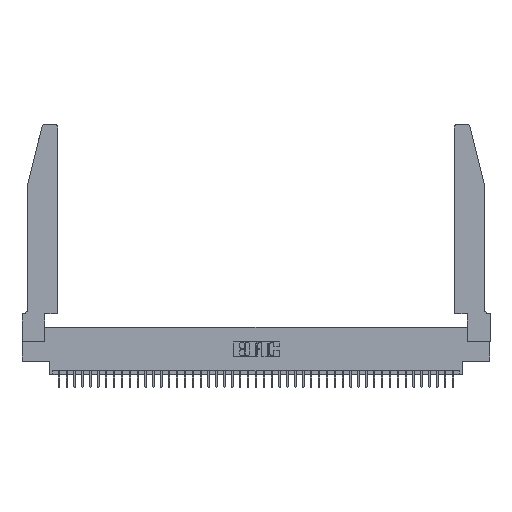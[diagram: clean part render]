
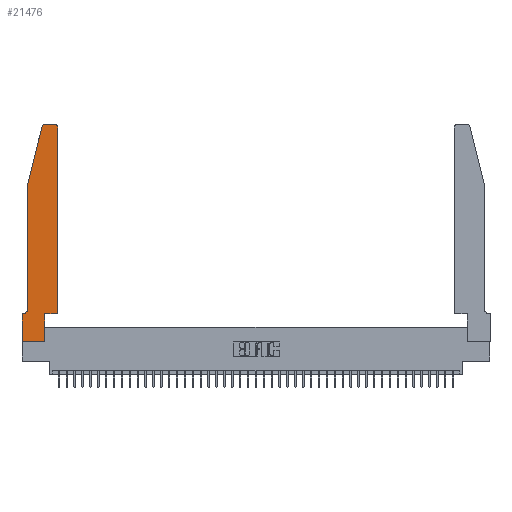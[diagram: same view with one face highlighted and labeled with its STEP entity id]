
A CAD part, top view. The second image highlights one B-rep face of the part: STEP entity #21476.
In plain terms, the highlighted planar face has unit normal (0, 0, 1).
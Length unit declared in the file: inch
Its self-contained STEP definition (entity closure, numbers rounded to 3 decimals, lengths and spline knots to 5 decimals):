
#201 = CARTESIAN_POINT ( 'NONE',  ( 0., 0.35, 0.37 ) ) ;
#630 = FACE_OUTER_BOUND ( 'NONE', #7524, .T. ) ;
#2480 = CARTESIAN_POINT ( 'NONE',  ( 0.4505, 0.35, 0.37 ) ) ;
#2744 = CARTESIAN_POINT ( 'NONE',  ( 0.0755, 2., 0.37 ) ) ;
#3392 = VECTOR ( 'NONE', #34415, 39.37008 ) ;
#3431 = VERTEX_POINT ( 'NONE', #37091 ) ;
#3990 = DIRECTION ( 'NONE',  ( 0., 1., 0. ) ) ;
#4061 = ORIENTED_EDGE ( 'NONE', *, *, #27604, .T. ) ;
#4428 = CARTESIAN_POINT ( 'NONE',  ( 0.4205, 2.75, 0.37 ) ) ;
#4953 = EDGE_CURVE ( 'NONE', #30414, #35835, #20170, .T. ) ;
#5195 = AXIS2_PLACEMENT_3D ( 'NONE', #39839, #42639, #13471 ) ;
#5774 = VECTOR ( 'NONE', #9943, 39.37008 ) ;
#6065 = VECTOR ( 'NONE', #11434, 39.37008 ) ;
#6273 = CARTESIAN_POINT ( 'NONE',  ( 0.2605, 2.75, 0.37 ) ) ;
#6941 = DIRECTION ( 'NONE',  ( 0., 0., 1. ) ) ;
#7218 = PLANE ( 'NONE',  #25998 ) ;
#7524 = EDGE_LOOP ( 'NONE', ( #34817, #4061, #43095, #39921, #35769, #30388, #33213, #10723, #20108, #25203, #20987, #14579 ) ) ;
#7546 = VERTEX_POINT ( 'NONE', #34997 ) ;
#8217 = LINE ( 'NONE', #36233, #42157 ) ;
#8268 = CARTESIAN_POINT ( 'NONE',  ( 0.4505, 2.72, 0.37 ) ) ;
#8286 = CIRCLE ( 'NONE', #5195, 0.03 ) ;
#9338 = DIRECTION ( 'NONE',  ( 0., 0., -1. ) ) ;
#9943 = DIRECTION ( 'NONE',  ( -0.239, -0.971, 0. ) ) ;
#10118 = VERTEX_POINT ( 'NONE', #12332 ) ;
#10639 = DIRECTION ( 'NONE',  ( 0., 1., 0. ) ) ;
#10723 = ORIENTED_EDGE ( 'NONE', *, *, #36089, .T. ) ;
#10824 = VERTEX_POINT ( 'NONE', #27825 ) ;
#11266 = CARTESIAN_POINT ( 'NONE',  ( 0.4505, 0.35, 0.37 ) ) ;
#11434 = DIRECTION ( 'NONE',  ( 0., -1., 0. ) ) ;
#11556 = LINE ( 'NONE', #6273, #28538 ) ;
#12150 = VERTEX_POINT ( 'NONE', #41210 ) ;
#12332 = CARTESIAN_POINT ( 'NONE',  ( 0.0755, 2., 0.37 ) ) ;
#12453 = EDGE_CURVE ( 'NONE', #40874, #32101, #20290, .T. ) ;
#13342 = CARTESIAN_POINT ( 'NONE',  ( 0.284, 2.75, 0.37 ) ) ;
#13358 = VECTOR ( 'NONE', #3990, 39.37008 ) ;
#13471 = DIRECTION ( 'NONE',  ( 1., 0., 0. ) ) ;
#14579 = ORIENTED_EDGE ( 'NONE', *, *, #4953, .T. ) ;
#15355 = EDGE_CURVE ( 'NONE', #35835, #32494, #11556, .T. ) ;
#15443 = VERTEX_POINT ( 'NONE', #24519 ) ;
#15636 = DIRECTION ( 'NONE',  ( -1., 0., 0. ) ) ;
#16541 = DIRECTION ( 'NONE',  ( -1., 0., 0. ) ) ;
#17772 = EDGE_CURVE ( 'NONE', #12150, #7546, #37866, .T. ) ;
#19574 = DIRECTION ( 'NONE',  ( 0., 0., 1. ) ) ;
#20108 = ORIENTED_EDGE ( 'NONE', *, *, #32672, .T. ) ;
#20170 = CIRCLE ( 'NONE', #40223, 0.03 ) ;
#20290 = CIRCLE ( 'NONE', #42739, 0.07 ) ;
#20987 = ORIENTED_EDGE ( 'NONE', *, *, #30800, .T. ) ;
#21420 = CARTESIAN_POINT ( 'NONE',  ( 0., 0., 0.37 ) ) ;
#21476 = ADVANCED_FACE ( 'NONE', ( #630 ), #7218, .T. ) ;
#22275 = EDGE_CURVE ( 'NONE', #3431, #10118, #37080, .T. ) ;
#23863 = CARTESIAN_POINT ( 'NONE',  ( 0.4505, 0.35, 0.37 ) ) ;
#24519 = CARTESIAN_POINT ( 'NONE',  ( 0.2865, 0., 0.37 ) ) ;
#25106 = CARTESIAN_POINT ( 'NONE',  ( 0.0055, 0.35, 0.37 ) ) ;
#25203 = ORIENTED_EDGE ( 'NONE', *, *, #31127, .T. ) ;
#25998 = AXIS2_PLACEMENT_3D ( 'NONE', #201, #6941, #27710 ) ;
#27604 = EDGE_CURVE ( 'NONE', #32494, #3431, #8286, .T. ) ;
#27705 = CARTESIAN_POINT ( 'NONE',  ( 0.2865, 0.35, 0.37 ) ) ;
#27710 = DIRECTION ( 'NONE',  ( 1., 0., 0. ) ) ;
#27781 = CARTESIAN_POINT ( 'NONE',  ( 0.0755, 0.35, 0.37 ) ) ;
#27825 = CARTESIAN_POINT ( 'NONE',  ( 0.2865, 0.35, 0.37 ) ) ;
#28538 = VECTOR ( 'NONE', #16541, 39.37008 ) ;
#29349 = LINE ( 'NONE', #33690, #3392 ) ;
#29489 = EDGE_CURVE ( 'NONE', #10118, #40874, #29349, .T. ) ;
#29608 = DIRECTION ( 'NONE',  ( 1., 0., 0. ) ) ;
#29638 = CARTESIAN_POINT ( 'NONE',  ( 0.0055, 0.42, 0.37 ) ) ;
#30388 = ORIENTED_EDGE ( 'NONE', *, *, #38103, .T. ) ;
#30414 = VERTEX_POINT ( 'NONE', #8268 ) ;
#30800 = EDGE_CURVE ( 'NONE', #42781, #30414, #34586, .T. ) ;
#31127 = EDGE_CURVE ( 'NONE', #10824, #42781, #33984, .T. ) ;
#31347 = LINE ( 'NONE', #27705, #42488 ) ;
#32101 = VERTEX_POINT ( 'NONE', #25106 ) ;
#32494 = VERTEX_POINT ( 'NONE', #13342 ) ;
#32672 = EDGE_CURVE ( 'NONE', #15443, #10824, #31347, .T. ) ;
#32927 = VECTOR ( 'NONE', #36388, 39.37008 ) ;
#33071 = VECTOR ( 'NONE', #37423, 39.37008 ) ;
#33213 = ORIENTED_EDGE ( 'NONE', *, *, #17772, .T. ) ;
#33690 = CARTESIAN_POINT ( 'NONE',  ( 0.0755, 2., 0.37 ) ) ;
#33984 = LINE ( 'NONE', #2480, #32927 ) ;
#34415 = DIRECTION ( 'NONE',  ( 0., -1., 0. ) ) ;
#34586 = LINE ( 'NONE', #23863, #13358 ) ;
#34817 = ORIENTED_EDGE ( 'NONE', *, *, #15355, .T. ) ;
#34997 = CARTESIAN_POINT ( 'NONE',  ( 0., 0., 0.37 ) ) ;
#35700 = LINE ( 'NONE', #27781, #33071 ) ;
#35769 = ORIENTED_EDGE ( 'NONE', *, *, #12453, .T. ) ;
#35835 = VERTEX_POINT ( 'NONE', #4428 ) ;
#36089 = EDGE_CURVE ( 'NONE', #7546, #15443, #8217, .T. ) ;
#36233 = CARTESIAN_POINT ( 'NONE',  ( 0., 0., 0.37 ) ) ;
#36388 = DIRECTION ( 'NONE',  ( 1., 0., 0. ) ) ;
#36759 = CARTESIAN_POINT ( 'NONE',  ( 0.4205, 2.72, 0.37 ) ) ;
#37080 = LINE ( 'NONE', #2744, #5774 ) ;
#37091 = CARTESIAN_POINT ( 'NONE',  ( 0.25487, 2.72718, 0.37 ) ) ;
#37423 = DIRECTION ( 'NONE',  ( -1., 0., 0. ) ) ;
#37866 = LINE ( 'NONE', #21420, #6065 ) ;
#38103 = EDGE_CURVE ( 'NONE', #32101, #12150, #35700, .T. ) ;
#39839 = CARTESIAN_POINT ( 'NONE',  ( 0.284, 2.72, 0.37 ) ) ;
#39921 = ORIENTED_EDGE ( 'NONE', *, *, #29489, .T. ) ;
#40223 = AXIS2_PLACEMENT_3D ( 'NONE', #36759, #19574, #29608 ) ;
#40874 = VERTEX_POINT ( 'NONE', #41337 ) ;
#41210 = CARTESIAN_POINT ( 'NONE',  ( 0., 0.35, 0.37 ) ) ;
#41337 = CARTESIAN_POINT ( 'NONE',  ( 0.0755, 0.42, 0.37 ) ) ;
#42157 = VECTOR ( 'NONE', #43448, 39.37008 ) ;
#42488 = VECTOR ( 'NONE', #10639, 39.37008 ) ;
#42639 = DIRECTION ( 'NONE',  ( 0., 0., 1. ) ) ;
#42739 = AXIS2_PLACEMENT_3D ( 'NONE', #29638, #9338, #15636 ) ;
#42781 = VERTEX_POINT ( 'NONE', #11266 ) ;
#43095 = ORIENTED_EDGE ( 'NONE', *, *, #22275, .T. ) ;
#43448 = DIRECTION ( 'NONE',  ( 1., 0., 0. ) ) ;
